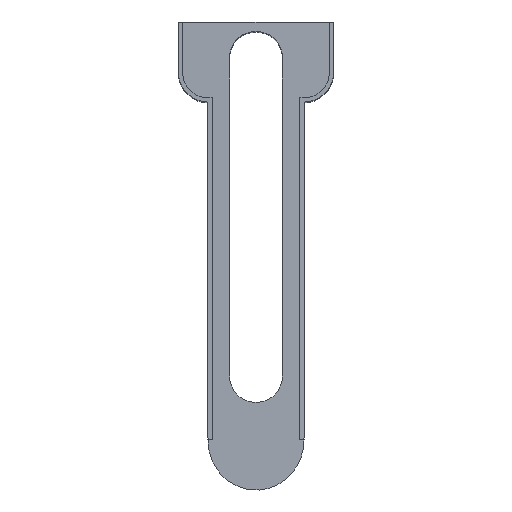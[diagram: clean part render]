
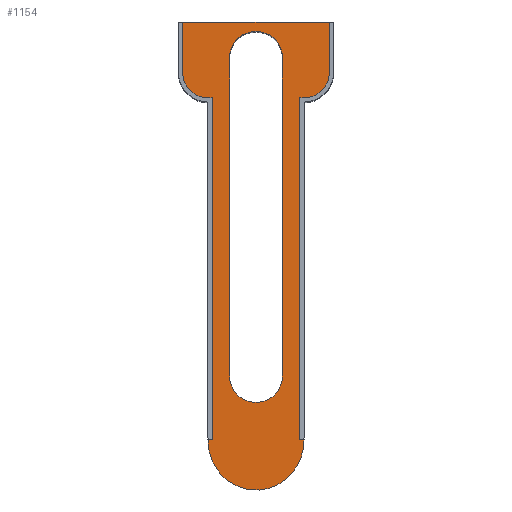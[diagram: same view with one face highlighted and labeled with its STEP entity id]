
A CAD part, top view. The second image highlights one B-rep face of the part: STEP entity #1154.
In plain terms, the highlighted planar face has unit normal (0, 0, 1).
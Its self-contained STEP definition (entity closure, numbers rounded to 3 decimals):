
#31 = AXIS2_PLACEMENT_3D ( 'NONE', #3343, #3226, #3448 ) ;
#49 = DIRECTION ( 'NONE',  ( 0., 0., -1. ) ) ;
#59 = CARTESIAN_POINT ( 'NONE',  ( -97.237, 35.875, 65.971 ) ) ;
#64 = DIRECTION ( 'NONE',  ( 1., 0., 0. ) ) ;
#68 = DIRECTION ( 'NONE',  ( 1., 0., 0. ) ) ;
#69 = DIRECTION ( 'NONE',  ( 0., 0., 1. ) ) ;
#76 = CARTESIAN_POINT ( 'NONE',  ( -108.747, 32.37, 65.971 ) ) ;
#87 = CARTESIAN_POINT ( 'NONE',  ( -107.747, 125.05, 65.971 ) ) ;
#95 = DIRECTION ( 'NONE',  ( 0., -1., 0. ) ) ;
#110 = CARTESIAN_POINT ( 'NONE',  ( -114.804, 125.05, 65.971 ) ) ;
#120 = DIRECTION ( 'NONE',  ( 0., -1., 0. ) ) ;
#121 = DIRECTION ( 'NONE',  ( 1., 0., 0. ) ) ;
#126 = DIRECTION ( 'NONE',  ( 0., 0., 1. ) ) ;
#131 = CARTESIAN_POINT ( 'NONE',  ( -85.728, 32.37, 65.971 ) ) ;
#133 = DIRECTION ( 'NONE',  ( 0., -1., 0. ) ) ;
#136 = CARTESIAN_POINT ( 'NONE',  ( -79.671, 125.05, 65.971 ) ) ;
#151 = DIRECTION ( 'NONE',  ( 0., -1., 0. ) ) ;
#155 = LINE ( 'NONE', #110, #2479 ) ;
#165 = CARTESIAN_POINT ( 'NONE',  ( -86.728, 125.05, 65.971 ) ) ;
#166 = CARTESIAN_POINT ( 'NONE',  ( -414.436, -55.678, 65.971 ) ) ;
#178 = DIRECTION ( 'NONE',  ( 1., 0., 0. ) ) ;
#185 = DIRECTION ( 'NONE',  ( 1., 0., 0. ) ) ;
#189 = CARTESIAN_POINT ( 'NONE',  ( -414.436, -55.678, 65.971 ) ) ;
#251 = VERTEX_POINT ( 'NONE', #1398 ) ;
#271 = LINE ( 'NONE', #165, #1956 ) ;
#278 = VERTEX_POINT ( 'NONE', #1327 ) ;
#305 = AXIS2_PLACEMENT_3D ( 'NONE', #76, #69, #64 ) ;
#339 = AXIS2_PLACEMENT_3D ( 'NONE', #131, #126, #121 ) ;
#392 = VECTOR ( 'NONE', #178, 1000. ) ;
#408 = CARTESIAN_POINT ( 'NONE',  ( -86.728, 26.396, 65.971 ) ) ;
#469 = CARTESIAN_POINT ( 'NONE',  ( -79.671, 44.49, 65.971 ) ) ;
#548 = EDGE_LOOP ( 'NONE', ( #1203, #1312, #2328, #2326, #2353, #1626, #1736, #1743, #1785, #1838 ) ) ;
#559 = CARTESIAN_POINT ( 'NONE',  ( -97.237, -46.674, 65.971 ) ) ;
#646 = VECTOR ( 'NONE', #1868, 1000. ) ;
#672 = EDGE_LOOP ( 'NONE', ( #1904, #1933, #1941, #1992, #2144, #2150 ) ) ;
#872 = EDGE_CURVE ( 'NONE', #1253, #251, #3127, .T. ) ;
#892 = EDGE_CURVE ( 'NONE', #1220, #278, #1244, .T. ) ;
#898 = EDGE_CURVE ( 'NONE', #3273, #1220, #271, .T. ) ;
#918 = EDGE_CURVE ( 'NONE', #3273, #2894, #2080, .T. ) ;
#925 = EDGE_CURVE ( 'NONE', #1078, #2894, #2413, .T. ) ;
#943 = AXIS2_PLACEMENT_3D ( 'NONE', #3182, #3177, #3175 ) ;
#955 = EDGE_CURVE ( 'NONE', #1452, #1591, #155, .T. ) ;
#962 = CARTESIAN_POINT ( 'NONE',  ( -90.887, 35.875, 65.971 ) ) ;
#978 = EDGE_CURVE ( 'NONE', #1591, #1271, #1010, .T. ) ;
#989 = EDGE_CURVE ( 'NONE', #1271, #251, #1128, .T. ) ;
#1010 = CIRCLE ( 'NONE', #305, 6.057 ) ;
#1034 = CARTESIAN_POINT ( 'NONE',  ( -97.237, 42.225, 65.971 ) ) ;
#1078 = VERTEX_POINT ( 'NONE', #469 ) ;
#1128 = LINE ( 'NONE', #87, #2924 ) ;
#1146 = VERTEX_POINT ( 'NONE', #3211 ) ;
#1154 = ADVANCED_FACE ( 'NONE', ( #2445, #1406 ), #3330, .T. ) ;
#1203 = ORIENTED_EDGE ( 'NONE', *, *, #872, .F. ) ;
#1220 = VERTEX_POINT ( 'NONE', #3153 ) ;
#1244 = LINE ( 'NONE', #166, #3068 ) ;
#1253 = VERTEX_POINT ( 'NONE', #3414 ) ;
#1271 = VERTEX_POINT ( 'NONE', #3113 ) ;
#1311 = EDGE_CURVE ( 'NONE', #1452, #1078, #1671, .T. ) ;
#1312 = ORIENTED_EDGE ( 'NONE', *, *, #2663, .F. ) ;
#1327 = CARTESIAN_POINT ( 'NONE',  ( -85.728, -55.678, 65.971 ) ) ;
#1330 = CARTESIAN_POINT ( 'NONE',  ( -103.587, 35.875, 65.971 ) ) ;
#1398 = CARTESIAN_POINT ( 'NONE',  ( -107.747, -55.678, 65.971 ) ) ;
#1406 = FACE_BOUND ( 'NONE', #672, .T. ) ;
#1452 = VERTEX_POINT ( 'NONE', #2160 ) ;
#1527 = CARTESIAN_POINT ( 'NONE',  ( -79.671, 32.37, 65.971 ) ) ;
#1591 = VERTEX_POINT ( 'NONE', #2257 ) ;
#1592 = CIRCLE ( 'NONE', #2231, 6.35 ) ;
#1611 = DIRECTION ( 'NONE',  ( 1., 0., 0. ) ) ;
#1617 = DIRECTION ( 'NONE',  ( 0., 0., -1. ) ) ;
#1621 = CARTESIAN_POINT ( 'NONE',  ( -97.237, 35.875, 65.971 ) ) ;
#1626 = ORIENTED_EDGE ( 'NONE', *, *, #925, .F. ) ;
#1671 = LINE ( 'NONE', #2236, #3395 ) ;
#1698 = LINE ( 'NONE', #1883, #646 ) ;
#1736 = ORIENTED_EDGE ( 'NONE', *, *, #1311, .F. ) ;
#1743 = ORIENTED_EDGE ( 'NONE', *, *, #955, .T. ) ;
#1765 = CIRCLE ( 'NONE', #3380, 6.35 ) ;
#1785 = ORIENTED_EDGE ( 'NONE', *, *, #978, .T. ) ;
#1807 = VERTEX_POINT ( 'NONE', #1330 ) ;
#1828 = DIRECTION ( 'NONE',  ( 1., 0., 0. ) ) ;
#1832 = DIRECTION ( 'NONE',  ( 0., 0., -1. ) ) ;
#1833 = CARTESIAN_POINT ( 'NONE',  ( -97.237, -40.325, 65.971 ) ) ;
#1837 = CARTESIAN_POINT ( 'NONE',  ( -103.587, 20.449, 65.971 ) ) ;
#1838 = ORIENTED_EDGE ( 'NONE', *, *, #989, .T. ) ;
#1847 = DIRECTION ( 'NONE',  ( 0., 1., 0. ) ) ;
#1868 = DIRECTION ( 'NONE',  ( 0., -1., 0. ) ) ;
#1883 = CARTESIAN_POINT ( 'NONE',  ( -90.887, 20.449, 65.971 ) ) ;
#1900 = VECTOR ( 'NONE', #133, 1000. ) ;
#1904 = ORIENTED_EDGE ( 'NONE', *, *, #2749, .T. ) ;
#1912 = CIRCLE ( 'NONE', #2402, 6.35 ) ;
#1933 = ORIENTED_EDGE ( 'NONE', *, *, #2045, .T. ) ;
#1941 = ORIENTED_EDGE ( 'NONE', *, *, #2768, .T. ) ;
#1956 = VECTOR ( 'NONE', #151, 1000. ) ;
#1963 = VERTEX_POINT ( 'NONE', #559 ) ;
#1977 = EDGE_CURVE ( 'NONE', #3063, #3079, #1765, .T. ) ;
#1979 = CARTESIAN_POINT ( 'NONE',  ( -108.747, -55.678, 65.971 ) ) ;
#1981 = CARTESIAN_POINT ( 'NONE',  ( -108.747, -79.728, 65.971 ) ) ;
#1992 = ORIENTED_EDGE ( 'NONE', *, *, #2773, .T. ) ;
#1997 = CARTESIAN_POINT ( 'NONE',  ( -85.728, -55.678, 65.971 ) ) ;
#2005 = CARTESIAN_POINT ( 'NONE',  ( -85.728, -79.728, 65.971 ) ) ;
#2045 = EDGE_CURVE ( 'NONE', #2464, #1963, #2687, .T. ) ;
#2080 = CIRCLE ( 'NONE', #339, 6.057 ) ;
#2144 = ORIENTED_EDGE ( 'NONE', *, *, #2860, .T. ) ;
#2150 = ORIENTED_EDGE ( 'NONE', *, *, #1977, .T. ) ;
#2160 = CARTESIAN_POINT ( 'NONE',  ( -114.804, 44.49, 65.971 ) ) ;
#2231 = AXIS2_PLACEMENT_3D ( 'NONE', #1833, #1832, #1828 ) ;
#2236 = CARTESIAN_POINT ( 'NONE',  ( -82.95, 44.49, 65.971 ) ) ;
#2257 = CARTESIAN_POINT ( 'NONE',  ( -114.804, 32.37, 65.971 ) ) ;
#2326 = ORIENTED_EDGE ( 'NONE', *, *, #898, .F. ) ;
#2328 = ORIENTED_EDGE ( 'NONE', *, *, #892, .F. ) ;
#2345 = CARTESIAN_POINT ( 'NONE',  ( -90.887, -40.325, 65.971 ) ) ;
#2353 = ORIENTED_EDGE ( 'NONE', *, *, #918, .T. ) ;
#2401 =( BOUNDED_CURVE ( )  B_SPLINE_CURVE ( 3, ( #1997, #2005, #1981, #1979 ),
 .UNSPECIFIED., .F., .T. ) 
 B_SPLINE_CURVE_WITH_KNOTS ( ( 4, 4 ),
 ( 4.712, 7.854 ),
 .UNSPECIFIED. ) 
 CURVE ( )  GEOMETRIC_REPRESENTATION_ITEM ( )  RATIONAL_B_SPLINE_CURVE ( ( 1., 0.333, 0.333, 1. ) ) 
 REPRESENTATION_ITEM ( '' )  );
#2402 = AXIS2_PLACEMENT_3D ( 'NONE', #1621, #1617, #1611 ) ;
#2413 = LINE ( 'NONE', #136, #1900 ) ;
#2445 = FACE_OUTER_BOUND ( 'NONE', #548, .T. ) ;
#2464 = VERTEX_POINT ( 'NONE', #2345 ) ;
#2479 = VECTOR ( 'NONE', #95, 1000. ) ;
#2663 = EDGE_CURVE ( 'NONE', #278, #1253, #2401, .T. ) ;
#2687 = CIRCLE ( 'NONE', #943, 6.35 ) ;
#2708 = VECTOR ( 'NONE', #1847, 1000. ) ;
#2749 = EDGE_CURVE ( 'NONE', #3079, #2464, #1698, .T. ) ;
#2768 = EDGE_CURVE ( 'NONE', #1963, #1146, #1592, .T. ) ;
#2773 = EDGE_CURVE ( 'NONE', #1146, #1807, #3278, .T. ) ;
#2860 = EDGE_CURVE ( 'NONE', #1807, #3063, #1912, .T. ) ;
#2894 = VERTEX_POINT ( 'NONE', #1527 ) ;
#2924 = VECTOR ( 'NONE', #120, 1000. ) ;
#3063 = VERTEX_POINT ( 'NONE', #1034 ) ;
#3068 = VECTOR ( 'NONE', #185, 1000. ) ;
#3079 = VERTEX_POINT ( 'NONE', #962 ) ;
#3113 = CARTESIAN_POINT ( 'NONE',  ( -107.747, 26.396, 65.971 ) ) ;
#3127 = LINE ( 'NONE', #189, #392 ) ;
#3153 = CARTESIAN_POINT ( 'NONE',  ( -86.728, -55.678, 65.971 ) ) ;
#3175 = DIRECTION ( 'NONE',  ( 1., 0., 0. ) ) ;
#3177 = DIRECTION ( 'NONE',  ( 0., 0., -1. ) ) ;
#3182 = CARTESIAN_POINT ( 'NONE',  ( -97.237, -40.325, 65.971 ) ) ;
#3211 = CARTESIAN_POINT ( 'NONE',  ( -103.587, -40.325, 65.971 ) ) ;
#3226 = DIRECTION ( 'NONE',  ( 0., 0., 1. ) ) ;
#3273 = VERTEX_POINT ( 'NONE', #408 ) ;
#3278 = LINE ( 'NONE', #1837, #2708 ) ;
#3330 = PLANE ( 'NONE',  #31 ) ;
#3343 = CARTESIAN_POINT ( 'NONE',  ( -414.436, 125.05, 65.971 ) ) ;
#3380 = AXIS2_PLACEMENT_3D ( 'NONE', #59, #49, #68 ) ;
#3388 = DIRECTION ( 'NONE',  ( 1., 0., 0. ) ) ;
#3395 = VECTOR ( 'NONE', #3388, 1000. ) ;
#3414 = CARTESIAN_POINT ( 'NONE',  ( -108.747, -55.678, 65.971 ) ) ;
#3448 = DIRECTION ( 'NONE',  ( 1., 0., 0. ) ) ;
